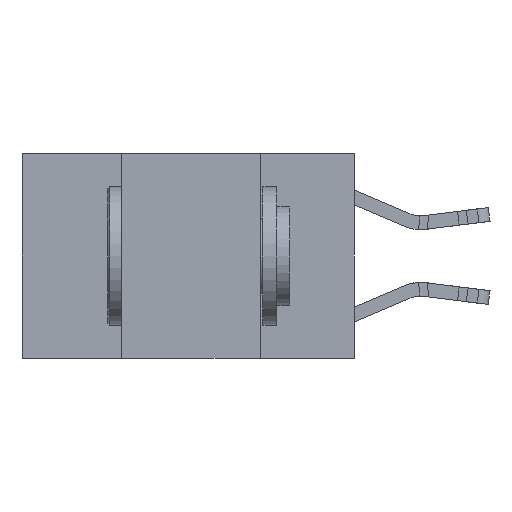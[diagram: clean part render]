
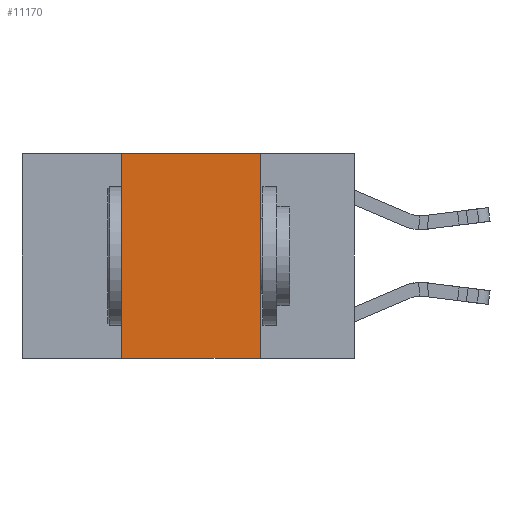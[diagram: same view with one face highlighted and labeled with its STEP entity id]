
A CAD part, left-side view. The second image highlights one B-rep face of the part: STEP entity #11170.
In plain terms, the highlighted planar face has unit normal (-1, 0, 0).
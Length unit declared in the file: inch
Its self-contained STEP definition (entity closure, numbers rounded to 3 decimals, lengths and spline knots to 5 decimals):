
#16 = VECTOR ( 'NONE', #23685, 39.37008 ) ;
#1443 = ORIENTED_EDGE ( 'NONE', *, *, #26159, .F. ) ;
#3286 = EDGE_CURVE ( 'NONE', #28286, #13162, #8979, .T. ) ;
#4207 = EDGE_CURVE ( 'NONE', #29576, #13162, #18571, .T. ) ;
#4376 = CARTESIAN_POINT ( 'NONE',  ( 0., 0.6, 0. ) ) ;
#4403 = EDGE_LOOP ( 'NONE', ( #24500, #19811, #1443, #11451 ) ) ;
#4902 = DIRECTION ( 'NONE',  ( 0., 0., -1. ) ) ;
#5841 = CARTESIAN_POINT ( 'NONE',  ( 0., 0.17, 0. ) ) ;
#6873 = EDGE_CURVE ( 'NONE', #27532, #28286, #16285, .T. ) ;
#7154 = CARTESIAN_POINT ( 'NONE',  ( 0., 0.6, -0.37 ) ) ;
#8979 = LINE ( 'NONE', #16945, #22352 ) ;
#9282 = CARTESIAN_POINT ( 'NONE',  ( 0., 0.17, -0.37 ) ) ;
#9315 = FACE_OUTER_BOUND ( 'NONE', #4403, .T. ) ;
#9461 = CARTESIAN_POINT ( 'NONE',  ( 0., 0.42, 0. ) ) ;
#9916 = DIRECTION ( 'NONE',  ( 0., -1., 0. ) ) ;
#11170 = ADVANCED_FACE ( 'NONE', ( #9315 ), #14688, .F. ) ;
#11451 = ORIENTED_EDGE ( 'NONE', *, *, #4207, .T. ) ;
#11725 = AXIS2_PLACEMENT_3D ( 'NONE', #28774, #14393, #19015 ) ;
#12961 = CARTESIAN_POINT ( 'NONE',  ( 0., 0.42, -0.37 ) ) ;
#13162 = VERTEX_POINT ( 'NONE', #9282 ) ;
#14393 = DIRECTION ( 'NONE',  ( 1., 0., 0. ) ) ;
#14688 = PLANE ( 'NONE',  #11725 ) ;
#15628 = LINE ( 'NONE', #25057, #16403 ) ;
#16285 = LINE ( 'NONE', #4376, #21153 ) ;
#16403 = VECTOR ( 'NONE', #27231, 39.37008 ) ;
#16945 = CARTESIAN_POINT ( 'NONE',  ( 0., 0.17, 0. ) ) ;
#18571 = LINE ( 'NONE', #7154, #16 ) ;
#19015 = DIRECTION ( 'NONE',  ( 0., 0., -1. ) ) ;
#19811 = ORIENTED_EDGE ( 'NONE', *, *, #6873, .F. ) ;
#21153 = VECTOR ( 'NONE', #9916, 39.37008 ) ;
#22352 = VECTOR ( 'NONE', #4902, 39.37008 ) ;
#23685 = DIRECTION ( 'NONE',  ( 0., -1., 0. ) ) ;
#24500 = ORIENTED_EDGE ( 'NONE', *, *, #3286, .F. ) ;
#25057 = CARTESIAN_POINT ( 'NONE',  ( 0., 0.42, 0. ) ) ;
#26159 = EDGE_CURVE ( 'NONE', #29576, #27532, #15628, .T. ) ;
#27231 = DIRECTION ( 'NONE',  ( 0., 0., 1. ) ) ;
#27532 = VERTEX_POINT ( 'NONE', #9461 ) ;
#28286 = VERTEX_POINT ( 'NONE', #5841 ) ;
#28774 = CARTESIAN_POINT ( 'NONE',  ( 0., 0.6, 0. ) ) ;
#29576 = VERTEX_POINT ( 'NONE', #12961 ) ;
